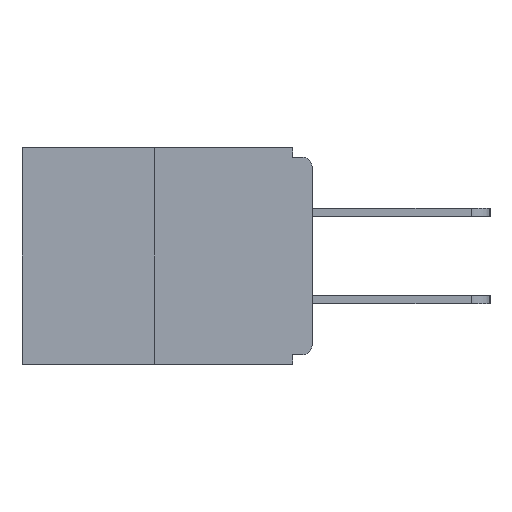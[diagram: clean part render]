
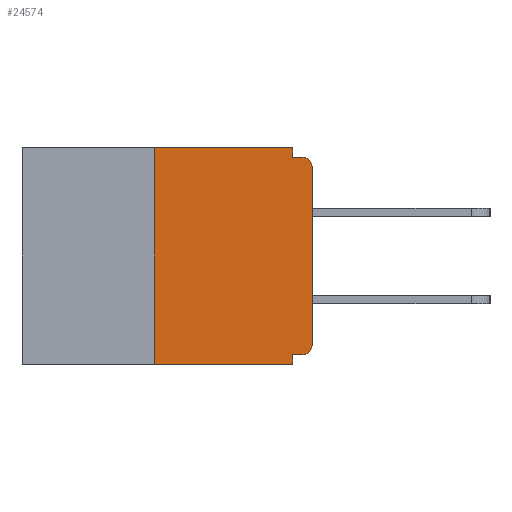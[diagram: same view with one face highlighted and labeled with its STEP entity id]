
A CAD part, left-side view. The second image highlights one B-rep face of the part: STEP entity #24574.
In plain terms, the highlighted planar face has unit normal (-1, 0, 0).
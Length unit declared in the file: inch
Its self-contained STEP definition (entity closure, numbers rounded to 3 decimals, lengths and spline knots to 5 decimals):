
#513 = VECTOR ( 'NONE', #20753, 39.37008 ) ;
#649 = VECTOR ( 'NONE', #4253, 39.37008 ) ;
#1291 = CARTESIAN_POINT ( 'NONE',  ( 0., 0.46, -0.343 ) ) ;
#1448 = CARTESIAN_POINT ( 'NONE',  ( 0., 0., -0.015 ) ) ;
#1794 = ORIENTED_EDGE ( 'NONE', *, *, #20732, .F. ) ;
#3100 = LINE ( 'NONE', #13872, #14347 ) ;
#3278 = DIRECTION ( 'NONE',  ( 0., 1., 0. ) ) ;
#3636 = ORIENTED_EDGE ( 'NONE', *, *, #8812, .F. ) ;
#3654 = LINE ( 'NONE', #18890, #21852 ) ;
#3701 = LINE ( 'NONE', #14318, #9895 ) ;
#3844 = CARTESIAN_POINT ( 'NONE',  ( 0., 0.25, 0. ) ) ;
#4253 = DIRECTION ( 'NONE',  ( 0., 0., 1. ) ) ;
#4325 = CARTESIAN_POINT ( 'NONE',  ( 0., 0., -0.313 ) ) ;
#4485 = VERTEX_POINT ( 'NONE', #7072 ) ;
#4496 = EDGE_CURVE ( 'NONE', #25735, #20845, #15332, .T. ) ;
#4724 = DIRECTION ( 'NONE',  ( 0., 0., 1. ) ) ;
#4873 = ORIENTED_EDGE ( 'NONE', *, *, #18161, .F. ) ;
#4874 = CARTESIAN_POINT ( 'NONE',  ( 0., 0.015, -0.03 ) ) ;
#4880 = DIRECTION ( 'NONE',  ( 0., -1., 0. ) ) ;
#5423 = ORIENTED_EDGE ( 'NONE', *, *, #4496, .T. ) ;
#5668 = DIRECTION ( 'NONE',  ( 0., 0., -1. ) ) ;
#6653 = VECTOR ( 'NONE', #22703, 39.37008 ) ;
#7072 = CARTESIAN_POINT ( 'NONE',  ( 0., 0.031, -0.015 ) ) ;
#7312 = CARTESIAN_POINT ( 'NONE',  ( 0., 0.031, -0.328 ) ) ;
#7597 = VERTEX_POINT ( 'NONE', #21275 ) ;
#8194 = ORIENTED_EDGE ( 'NONE', *, *, #24426, .F. ) ;
#8812 = EDGE_CURVE ( 'NONE', #12731, #26876, #12507, .T. ) ;
#9192 = DIRECTION ( 'NONE',  ( 0., 0., -1. ) ) ;
#9715 = AXIS2_PLACEMENT_3D ( 'NONE', #4874, #21800, #9192 ) ;
#9895 = VECTOR ( 'NONE', #3278, 39.37008 ) ;
#10070 = CARTESIAN_POINT ( 'NONE',  ( 0., 0.015, -0.313 ) ) ;
#10833 = VERTEX_POINT ( 'NONE', #22092 ) ;
#11947 = LINE ( 'NONE', #1448, #513 ) ;
#12507 = LINE ( 'NONE', #3844, #649 ) ;
#12598 = DIRECTION ( 'NONE',  ( 0., 0., -1. ) ) ;
#12731 = VERTEX_POINT ( 'NONE', #26841 ) ;
#13282 = CIRCLE ( 'NONE', #9715, 0.015 ) ;
#13285 = AXIS2_PLACEMENT_3D ( 'NONE', #10070, #18601, #21128 ) ;
#13851 = CARTESIAN_POINT ( 'NONE',  ( 0., 0.25, 0. ) ) ;
#13872 = CARTESIAN_POINT ( 'NONE',  ( 0., 0.031, 0. ) ) ;
#14053 = EDGE_CURVE ( 'NONE', #21724, #4485, #3100, .T. ) ;
#14058 = FACE_OUTER_BOUND ( 'NONE', #15919, .T. ) ;
#14318 = CARTESIAN_POINT ( 'NONE',  ( 0., 0., -0.328 ) ) ;
#14347 = VECTOR ( 'NONE', #21849, 39.37008 ) ;
#15034 = ORIENTED_EDGE ( 'NONE', *, *, #14053, .F. ) ;
#15332 = LINE ( 'NONE', #23882, #21702 ) ;
#15919 = EDGE_LOOP ( 'NONE', ( #8194, #3636, #20356, #4873, #16994, #23648, #5423, #18190, #1794, #15034 ) ) ;
#15964 = CIRCLE ( 'NONE', #13285, 0.015 ) ;
#16135 = VERTEX_POINT ( 'NONE', #7312 ) ;
#16968 = CARTESIAN_POINT ( 'NONE',  ( 0., 0., -0.03 ) ) ;
#16994 = ORIENTED_EDGE ( 'NONE', *, *, #20713, .F. ) ;
#17501 = EDGE_CURVE ( 'NONE', #12731, #10833, #20456, .T. ) ;
#17596 = LINE ( 'NONE', #24042, #20827 ) ;
#17821 = PLANE ( 'NONE',  #21809 ) ;
#18161 = EDGE_CURVE ( 'NONE', #16135, #10833, #3654, .T. ) ;
#18190 = ORIENTED_EDGE ( 'NONE', *, *, #27210, .T. ) ;
#18601 = DIRECTION ( 'NONE',  ( -1., 0., 0. ) ) ;
#18890 = CARTESIAN_POINT ( 'NONE',  ( 0., 0.031, -0.343 ) ) ;
#19798 = CARTESIAN_POINT ( 'NONE',  ( 0., 0.031, 0. ) ) ;
#20356 = ORIENTED_EDGE ( 'NONE', *, *, #17501, .T. ) ;
#20456 = LINE ( 'NONE', #1291, #6653 ) ;
#20713 = EDGE_CURVE ( 'NONE', #25089, #16135, #3701, .T. ) ;
#20732 = EDGE_CURVE ( 'NONE', #4485, #7597, #11947, .T. ) ;
#20753 = DIRECTION ( 'NONE',  ( 0., -1., 0. ) ) ;
#20827 = VECTOR ( 'NONE', #4880, 39.37008 ) ;
#20845 = VERTEX_POINT ( 'NONE', #16968 ) ;
#21128 = DIRECTION ( 'NONE',  ( 0., 0., -1. ) ) ;
#21275 = CARTESIAN_POINT ( 'NONE',  ( 0., 0.015, -0.015 ) ) ;
#21702 = VECTOR ( 'NONE', #4724, 39.37008 ) ;
#21724 = VERTEX_POINT ( 'NONE', #19798 ) ;
#21800 = DIRECTION ( 'NONE',  ( -1., 0., 0. ) ) ;
#21809 = AXIS2_PLACEMENT_3D ( 'NONE', #26374, #26793, #5668 ) ;
#21849 = DIRECTION ( 'NONE',  ( 0., 0., -1. ) ) ;
#21852 = VECTOR ( 'NONE', #12598, 39.37008 ) ;
#22092 = CARTESIAN_POINT ( 'NONE',  ( 0., 0.031, -0.343 ) ) ;
#22703 = DIRECTION ( 'NONE',  ( 0., -1., 0. ) ) ;
#22738 = CARTESIAN_POINT ( 'NONE',  ( 0., 0.015, -0.328 ) ) ;
#23648 = ORIENTED_EDGE ( 'NONE', *, *, #25438, .T. ) ;
#23882 = CARTESIAN_POINT ( 'NONE',  ( 0., 0., 0. ) ) ;
#24042 = CARTESIAN_POINT ( 'NONE',  ( 0., 0.46, 0. ) ) ;
#24426 = EDGE_CURVE ( 'NONE', #26876, #21724, #17596, .T. ) ;
#24574 = ADVANCED_FACE ( 'NONE', ( #14058 ), #17821, .F. ) ;
#25089 = VERTEX_POINT ( 'NONE', #22738 ) ;
#25438 = EDGE_CURVE ( 'NONE', #25089, #25735, #15964, .T. ) ;
#25735 = VERTEX_POINT ( 'NONE', #4325 ) ;
#26374 = CARTESIAN_POINT ( 'NONE',  ( 0., 0.46, 0. ) ) ;
#26793 = DIRECTION ( 'NONE',  ( 1., 0., 0. ) ) ;
#26841 = CARTESIAN_POINT ( 'NONE',  ( 0., 0.25, -0.343 ) ) ;
#26876 = VERTEX_POINT ( 'NONE', #13851 ) ;
#27210 = EDGE_CURVE ( 'NONE', #20845, #7597, #13282, .T. ) ;
